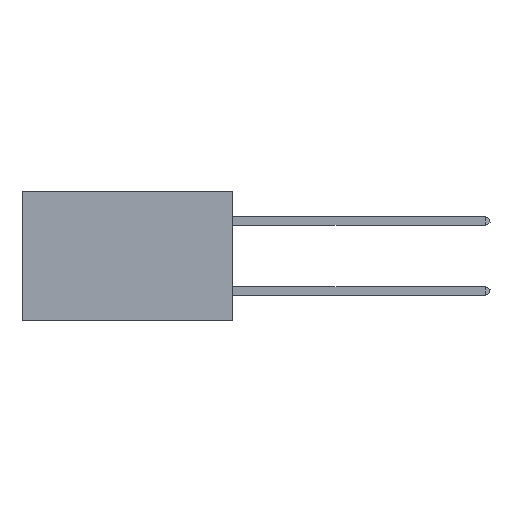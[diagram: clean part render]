
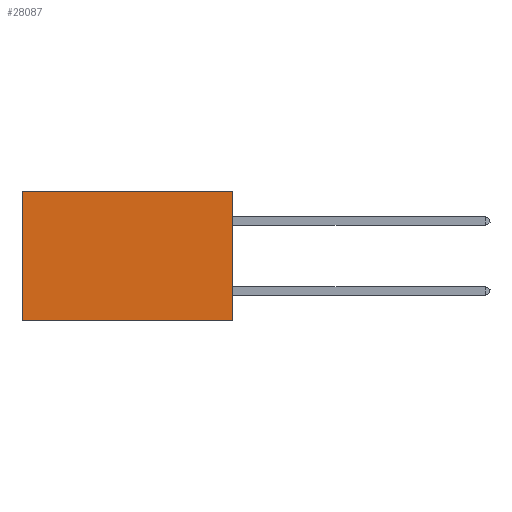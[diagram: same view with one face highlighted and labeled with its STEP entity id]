
A CAD part, left-side view. The second image highlights one B-rep face of the part: STEP entity #28087.
In plain terms, the highlighted planar face has unit normal (-1, 0, 0).
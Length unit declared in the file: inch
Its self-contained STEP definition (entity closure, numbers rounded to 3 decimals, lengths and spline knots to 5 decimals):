
#464 = EDGE_CURVE ( 'NONE', #34202, #914, #28043, .T. ) ;
#795 = CARTESIAN_POINT ( 'NONE',  ( 0.2875, 0., 0. ) ) ;
#914 = VERTEX_POINT ( 'NONE', #21876 ) ;
#1470 = VERTEX_POINT ( 'NONE', #1867 ) ;
#1867 = CARTESIAN_POINT ( 'NONE',  ( 0.2875, 0., 0. ) ) ;
#2006 = CARTESIAN_POINT ( 'NONE',  ( 0.2875, 0., -0.37 ) ) ;
#2787 = ORIENTED_EDGE ( 'NONE', *, *, #19039, .T. ) ;
#3315 = VECTOR ( 'NONE', #4132, 39.37008 ) ;
#4107 = ORIENTED_EDGE ( 'NONE', *, *, #25713, .F. ) ;
#4132 = DIRECTION ( 'NONE',  ( 0., 0., -1. ) ) ;
#5201 = VERTEX_POINT ( 'NONE', #21834 ) ;
#6372 = CARTESIAN_POINT ( 'NONE',  ( 0.2875, 0., 0. ) ) ;
#6812 = FACE_OUTER_BOUND ( 'NONE', #36739, .T. ) ;
#7316 = LINE ( 'NONE', #8124, #40422 ) ;
#8124 = CARTESIAN_POINT ( 'NONE',  ( 0.2875, 0.6, 0. ) ) ;
#9239 = ORIENTED_EDGE ( 'NONE', *, *, #25962, .T. ) ;
#10184 = DIRECTION ( 'NONE',  ( 0., 1., 0. ) ) ;
#11031 = AXIS2_PLACEMENT_3D ( 'NONE', #6372, #35276, #16192 ) ;
#12897 = PLANE ( 'NONE',  #11031 ) ;
#16192 = DIRECTION ( 'NONE',  ( 0., 0., -1. ) ) ;
#17968 = DIRECTION ( 'NONE',  ( 0., 0., -1. ) ) ;
#19039 = EDGE_CURVE ( 'NONE', #5201, #914, #7316, .T. ) ;
#20136 = ORIENTED_EDGE ( 'NONE', *, *, #464, .F. ) ;
#21834 = CARTESIAN_POINT ( 'NONE',  ( 0.2875, 0.6, 0. ) ) ;
#21876 = CARTESIAN_POINT ( 'NONE',  ( 0.2875, 0.6, -0.37 ) ) ;
#24733 = DIRECTION ( 'NONE',  ( 0., 1., 0. ) ) ;
#25713 = EDGE_CURVE ( 'NONE', #1470, #34202, #29095, .T. ) ;
#25962 = EDGE_CURVE ( 'NONE', #1470, #5201, #36121, .T. ) ;
#26280 = CARTESIAN_POINT ( 'NONE',  ( 0.2875, 0., -0.37 ) ) ;
#27708 = VECTOR ( 'NONE', #24733, 39.37008 ) ;
#28043 = LINE ( 'NONE', #26280, #29042 ) ;
#28087 = ADVANCED_FACE ( 'NONE', ( #6812 ), #12897, .F. ) ;
#29042 = VECTOR ( 'NONE', #10184, 39.37008 ) ;
#29095 = LINE ( 'NONE', #795, #3315 ) ;
#34197 = CARTESIAN_POINT ( 'NONE',  ( 0.2875, 0., 0. ) ) ;
#34202 = VERTEX_POINT ( 'NONE', #2006 ) ;
#35276 = DIRECTION ( 'NONE',  ( 1., 0., 0. ) ) ;
#36121 = LINE ( 'NONE', #34197, #27708 ) ;
#36739 = EDGE_LOOP ( 'NONE', ( #2787, #20136, #4107, #9239 ) ) ;
#40422 = VECTOR ( 'NONE', #17968, 39.37008 ) ;
